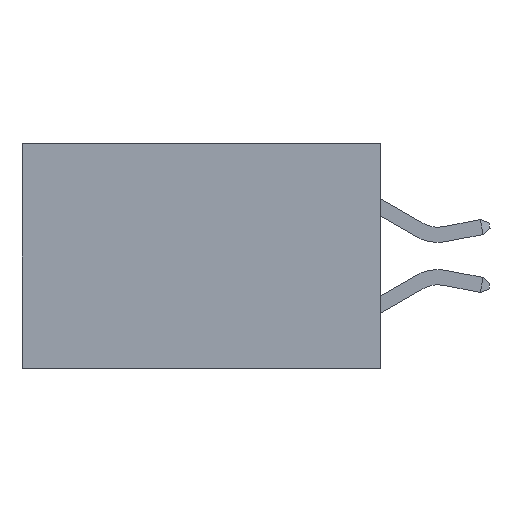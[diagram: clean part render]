
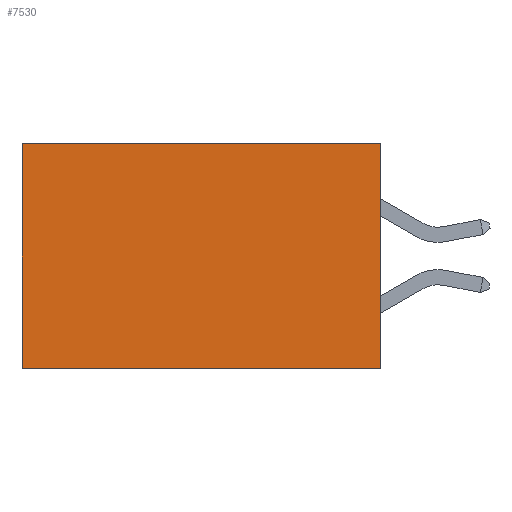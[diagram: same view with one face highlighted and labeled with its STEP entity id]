
A CAD part, left-side view. The second image highlights one B-rep face of the part: STEP entity #7530.
In plain terms, the highlighted planar face has unit normal (-1, 0, 0).
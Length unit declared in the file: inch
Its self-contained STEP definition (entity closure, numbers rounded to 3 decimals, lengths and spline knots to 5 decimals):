
#590 = VERTEX_POINT ( 'NONE', #10556 ) ;
#657 = CARTESIAN_POINT ( 'NONE',  ( 0.277, 0.59, -0.37 ) ) ;
#1062 = LINE ( 'NONE', #13380, #13383 ) ;
#1187 = EDGE_CURVE ( 'NONE', #27110, #15280, #1062, .T. ) ;
#1482 = CARTESIAN_POINT ( 'NONE',  ( 0.277, 0., 0. ) ) ;
#1798 = DIRECTION ( 'NONE',  ( 0., 0., -1. ) ) ;
#1883 = ORIENTED_EDGE ( 'NONE', *, *, #1187, .F. ) ;
#3826 = VECTOR ( 'NONE', #15659, 39.37008 ) ;
#5099 = CARTESIAN_POINT ( 'NONE',  ( 0.277, 0.59, -0.37 ) ) ;
#6672 = CARTESIAN_POINT ( 'NONE',  ( 0.277, 0., -0.37 ) ) ;
#6764 = VECTOR ( 'NONE', #24893, 39.37008 ) ;
#7530 = ADVANCED_FACE ( 'NONE', ( #11568 ), #14058, .F. ) ;
#7536 = LINE ( 'NONE', #657, #6764 ) ;
#10556 = CARTESIAN_POINT ( 'NONE',  ( 0.277, 0.59, 0. ) ) ;
#11281 = ORIENTED_EDGE ( 'NONE', *, *, #31329, .T. ) ;
#11568 = FACE_OUTER_BOUND ( 'NONE', #12290, .T. ) ;
#12290 = EDGE_LOOP ( 'NONE', ( #18527, #1883, #26508, #11281 ) ) ;
#13380 = CARTESIAN_POINT ( 'NONE',  ( 0.277, 0., -0.37 ) ) ;
#13383 = VECTOR ( 'NONE', #20221, 39.37008 ) ;
#14058 = PLANE ( 'NONE',  #14483 ) ;
#14434 = VECTOR ( 'NONE', #31391, 39.37008 ) ;
#14483 = AXIS2_PLACEMENT_3D ( 'NONE', #6672, #16491, #1798 ) ;
#15280 = VERTEX_POINT ( 'NONE', #5099 ) ;
#15659 = DIRECTION ( 'NONE',  ( 0., 1., 0. ) ) ;
#16491 = DIRECTION ( 'NONE',  ( 1., 0., 0. ) ) ;
#16953 = CARTESIAN_POINT ( 'NONE',  ( 0.277, 0., -0.37 ) ) ;
#18527 = ORIENTED_EDGE ( 'NONE', *, *, #23250, .T. ) ;
#19312 = CARTESIAN_POINT ( 'NONE',  ( 0.277, 0., -0.37 ) ) ;
#20221 = DIRECTION ( 'NONE',  ( 0., 1., 0. ) ) ;
#20468 = CARTESIAN_POINT ( 'NONE',  ( 0.277, 0., 0. ) ) ;
#20817 = LINE ( 'NONE', #19312, #14434 ) ;
#21587 = VERTEX_POINT ( 'NONE', #1482 ) ;
#22987 = EDGE_CURVE ( 'NONE', #21587, #27110, #20817, .T. ) ;
#23250 = EDGE_CURVE ( 'NONE', #590, #15280, #7536, .T. ) ;
#24893 = DIRECTION ( 'NONE',  ( 0., 0., -1. ) ) ;
#26508 = ORIENTED_EDGE ( 'NONE', *, *, #22987, .F. ) ;
#27110 = VERTEX_POINT ( 'NONE', #16953 ) ;
#29676 = LINE ( 'NONE', #20468, #3826 ) ;
#31329 = EDGE_CURVE ( 'NONE', #21587, #590, #29676, .T. ) ;
#31391 = DIRECTION ( 'NONE',  ( 0., 0., -1. ) ) ;
